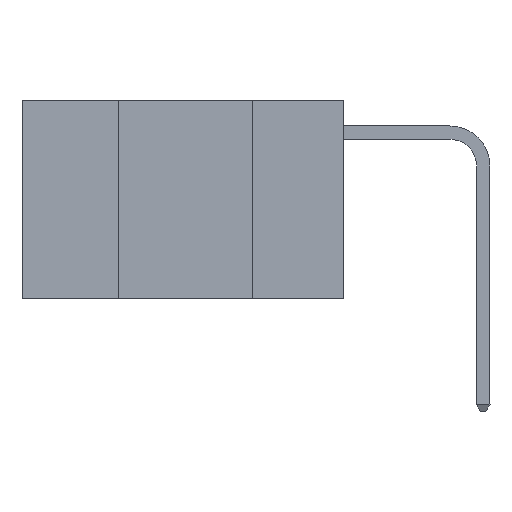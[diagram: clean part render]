
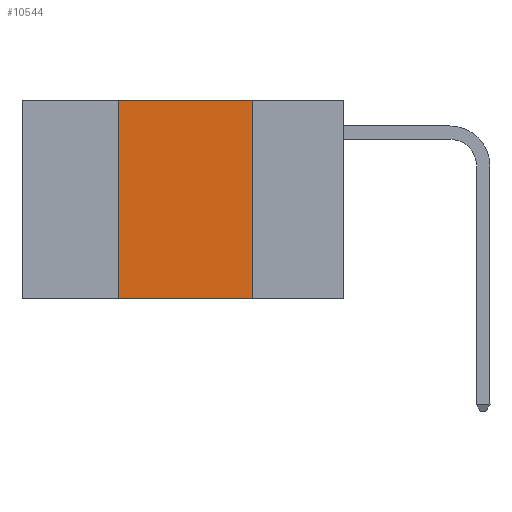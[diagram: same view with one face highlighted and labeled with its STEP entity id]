
A CAD part, left-side view. The second image highlights one B-rep face of the part: STEP entity #10544.
In plain terms, the highlighted planar face has unit normal (-1, 0, 0).
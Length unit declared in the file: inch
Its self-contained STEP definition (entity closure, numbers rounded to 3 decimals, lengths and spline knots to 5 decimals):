
#550 = VECTOR ( 'NONE', #13796, 39.37008 ) ;
#697 = LINE ( 'NONE', #3189, #5583 ) ;
#804 = AXIS2_PLACEMENT_3D ( 'NONE', #16235, #10761, #1284 ) ;
#1215 = CARTESIAN_POINT ( 'NONE',  ( 0., 0.42, -0.37 ) ) ;
#1284 = DIRECTION ( 'NONE',  ( 0., 0., -1. ) ) ;
#1394 = VERTEX_POINT ( 'NONE', #1215 ) ;
#2052 = ORIENTED_EDGE ( 'NONE', *, *, #6183, .T. ) ;
#2659 = VECTOR ( 'NONE', #4208, 39.37008 ) ;
#3189 = CARTESIAN_POINT ( 'NONE',  ( 0., 0.42, 0. ) ) ;
#3692 = EDGE_CURVE ( 'NONE', #10679, #6516, #10730, .T. ) ;
#4104 = VECTOR ( 'NONE', #9918, 39.37008 ) ;
#4208 = DIRECTION ( 'NONE',  ( 0., -1., 0. ) ) ;
#4521 = CARTESIAN_POINT ( 'NONE',  ( 0., 0.6, 0. ) ) ;
#4594 = VERTEX_POINT ( 'NONE', #11186 ) ;
#5260 = ORIENTED_EDGE ( 'NONE', *, *, #8391, .F. ) ;
#5457 = LINE ( 'NONE', #13571, #2659 ) ;
#5583 = VECTOR ( 'NONE', #11134, 39.37008 ) ;
#6183 = EDGE_CURVE ( 'NONE', #1394, #4594, #5457, .T. ) ;
#6248 = EDGE_LOOP ( 'NONE', ( #8257, #7225, #5260, #2052 ) ) ;
#6516 = VERTEX_POINT ( 'NONE', #10360 ) ;
#6799 = FACE_OUTER_BOUND ( 'NONE', #6248, .T. ) ;
#6850 = CARTESIAN_POINT ( 'NONE',  ( 0., 0.17, 0. ) ) ;
#7225 = ORIENTED_EDGE ( 'NONE', *, *, #3692, .F. ) ;
#8257 = ORIENTED_EDGE ( 'NONE', *, *, #10938, .F. ) ;
#8391 = EDGE_CURVE ( 'NONE', #1394, #10679, #697, .T. ) ;
#9457 = PLANE ( 'NONE',  #804 ) ;
#9918 = DIRECTION ( 'NONE',  ( 0., -1., 0. ) ) ;
#10360 = CARTESIAN_POINT ( 'NONE',  ( 0., 0.17, 0. ) ) ;
#10544 = ADVANCED_FACE ( 'NONE', ( #6799 ), #9457, .F. ) ;
#10679 = VERTEX_POINT ( 'NONE', #11192 ) ;
#10730 = LINE ( 'NONE', #4521, #4104 ) ;
#10761 = DIRECTION ( 'NONE',  ( 1., 0., 0. ) ) ;
#10938 = EDGE_CURVE ( 'NONE', #6516, #4594, #10982, .T. ) ;
#10982 = LINE ( 'NONE', #6850, #550 ) ;
#11134 = DIRECTION ( 'NONE',  ( 0., 0., 1. ) ) ;
#11186 = CARTESIAN_POINT ( 'NONE',  ( 0., 0.17, -0.37 ) ) ;
#11192 = CARTESIAN_POINT ( 'NONE',  ( 0., 0.42, 0. ) ) ;
#13571 = CARTESIAN_POINT ( 'NONE',  ( 0., 0.6, -0.37 ) ) ;
#13796 = DIRECTION ( 'NONE',  ( 0., 0., -1. ) ) ;
#16235 = CARTESIAN_POINT ( 'NONE',  ( 0., 0.6, 0. ) ) ;
